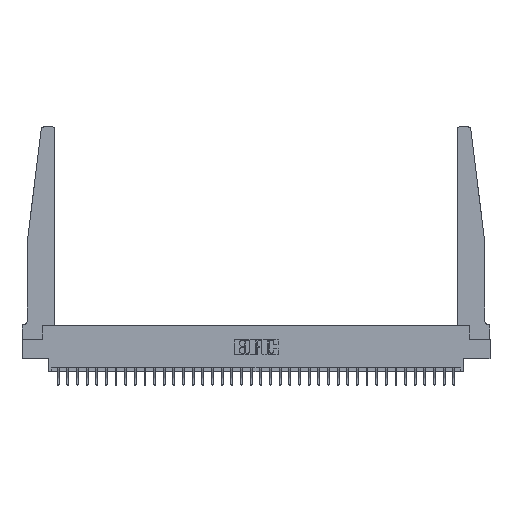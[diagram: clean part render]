
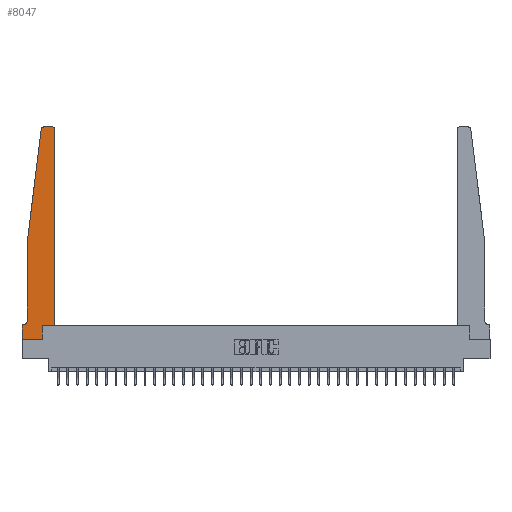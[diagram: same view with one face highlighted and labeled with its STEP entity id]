
A CAD part, top view. The second image highlights one B-rep face of the part: STEP entity #8047.
In plain terms, the highlighted planar face has unit normal (0, 0, 1).
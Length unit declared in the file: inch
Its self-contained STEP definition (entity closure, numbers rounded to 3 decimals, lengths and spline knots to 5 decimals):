
#39 = CARTESIAN_POINT ( 'NONE',  ( 0.015, 0.1875, 0.37 ) ) ;
#314 = CIRCLE ( 'NONE', #18942, 0.03 ) ;
#1138 = CARTESIAN_POINT ( 'NONE',  ( 0., 0., 0.37 ) ) ;
#1327 = CARTESIAN_POINT ( 'NONE',  ( 0.24675, 2.72367, 0.37 ) ) ;
#1437 = CARTESIAN_POINT ( 'NONE',  ( 0.25, 2.75, 0.37 ) ) ;
#2381 = DIRECTION ( 'NONE',  ( -1., 0., 0. ) ) ;
#2454 = CARTESIAN_POINT ( 'NONE',  ( 0., 0.1875, 0.37 ) ) ;
#2871 = CARTESIAN_POINT ( 'NONE',  ( 0.2605, 0.18, 0.37 ) ) ;
#2925 = ORIENTED_EDGE ( 'NONE', *, *, #31619, .T. ) ;
#3342 = VERTEX_POINT ( 'NONE', #1327 ) ;
#3439 = ORIENTED_EDGE ( 'NONE', *, *, #24675, .T. ) ;
#4040 = CARTESIAN_POINT ( 'NONE',  ( 0.425, 0.18, 0.37 ) ) ;
#4170 = ORIENTED_EDGE ( 'NONE', *, *, #29657, .T. ) ;
#4952 = VERTEX_POINT ( 'NONE', #29037 ) ;
#5104 = ORIENTED_EDGE ( 'NONE', *, *, #27729, .T. ) ;
#5352 = CARTESIAN_POINT ( 'NONE',  ( 0.015, 0.2375, 0.37 ) ) ;
#5631 = CARTESIAN_POINT ( 'NONE',  ( 0.065, 1.25, 0.37 ) ) ;
#5677 = AXIS2_PLACEMENT_3D ( 'NONE', #10539, #20381, #30613 ) ;
#5754 = CARTESIAN_POINT ( 'NONE',  ( 0.065, 1.25, 0.37 ) ) ;
#5912 = LINE ( 'NONE', #26119, #26464 ) ;
#6540 = LINE ( 'NONE', #4040, #9961 ) ;
#6696 = VECTOR ( 'NONE', #18986, 39.37008 ) ;
#6991 = VERTEX_POINT ( 'NONE', #2871 ) ;
#7453 = PLANE ( 'NONE',  #20711 ) ;
#7539 = VERTEX_POINT ( 'NONE', #30553 ) ;
#7604 = VECTOR ( 'NONE', #27082, 39.37008 ) ;
#7741 = VERTEX_POINT ( 'NONE', #18817 ) ;
#7951 = CARTESIAN_POINT ( 'NONE',  ( 0.425, 0.18, 0.37 ) ) ;
#7952 = ORIENTED_EDGE ( 'NONE', *, *, #28186, .T. ) ;
#8047 = ADVANCED_FACE ( 'NONE', ( #20122 ), #7453, .T. ) ;
#8212 = ORIENTED_EDGE ( 'NONE', *, *, #19629, .T. ) ;
#9096 = DIRECTION ( 'NONE',  ( 0., 0., 1. ) ) ;
#9371 = DIRECTION ( 'NONE',  ( 0., 1., 0. ) ) ;
#9961 = VECTOR ( 'NONE', #9371, 39.37008 ) ;
#10265 = ORIENTED_EDGE ( 'NONE', *, *, #20039, .T. ) ;
#10450 = VERTEX_POINT ( 'NONE', #32106 ) ;
#10491 = LINE ( 'NONE', #1138, #6696 ) ;
#10539 = CARTESIAN_POINT ( 'NONE',  ( 0.27653, 2.72, 0.37 ) ) ;
#11610 = DIRECTION ( 'NONE',  ( -1., 0., 0. ) ) ;
#12299 = VECTOR ( 'NONE', #2381, 39.37008 ) ;
#12859 = DIRECTION ( 'NONE',  ( 0., 0., -1. ) ) ;
#13132 = DIRECTION ( 'NONE',  ( 1., 0., 0. ) ) ;
#13327 = EDGE_CURVE ( 'NONE', #23776, #4952, #24910, .T. ) ;
#13438 = VERTEX_POINT ( 'NONE', #23059 ) ;
#13571 = ORIENTED_EDGE ( 'NONE', *, *, #19823, .T. ) ;
#13890 = CARTESIAN_POINT ( 'NONE',  ( 0., 0., 0.37 ) ) ;
#15115 = CARTESIAN_POINT ( 'NONE',  ( 0.27653, 2.75, 0.37 ) ) ;
#15221 = CARTESIAN_POINT ( 'NONE',  ( 0.065, 0.1875, 0.37 ) ) ;
#15334 = VERTEX_POINT ( 'NONE', #24056 ) ;
#16117 = VECTOR ( 'NONE', #11610, 39.37008 ) ;
#17402 = CARTESIAN_POINT ( 'NONE',  ( 0.2605, 0., 0.37 ) ) ;
#17425 = ORIENTED_EDGE ( 'NONE', *, *, #13327, .T. ) ;
#18127 = LINE ( 'NONE', #5631, #30673 ) ;
#18297 = DIRECTION ( 'NONE',  ( -0.122, -0.992, 0. ) ) ;
#18465 = LINE ( 'NONE', #7951, #22492 ) ;
#18539 = AXIS2_PLACEMENT_3D ( 'NONE', #5352, #12859, #30252 ) ;
#18580 = DIRECTION ( 'NONE',  ( 0., 1., 0. ) ) ;
#18817 = CARTESIAN_POINT ( 'NONE',  ( 0., 0., 0.37 ) ) ;
#18942 = AXIS2_PLACEMENT_3D ( 'NONE', #19432, #9096, #29997 ) ;
#18986 = DIRECTION ( 'NONE',  ( 0., -1., 0. ) ) ;
#19211 = LINE ( 'NONE', #13890, #7604 ) ;
#19432 = CARTESIAN_POINT ( 'NONE',  ( 0.395, 2.72, 0.37 ) ) ;
#19629 = EDGE_CURVE ( 'NONE', #6991, #7539, #18465, .T. ) ;
#19823 = EDGE_CURVE ( 'NONE', #10450, #30563, #24454, .T. ) ;
#20039 = EDGE_CURVE ( 'NONE', #15334, #13438, #25801, .T. ) ;
#20122 = FACE_OUTER_BOUND ( 'NONE', #27023, .T. ) ;
#20188 = VERTEX_POINT ( 'NONE', #17402 ) ;
#20381 = DIRECTION ( 'NONE',  ( 0., 0., 1. ) ) ;
#20651 = CIRCLE ( 'NONE', #18539, 0.05 ) ;
#20711 = AXIS2_PLACEMENT_3D ( 'NONE', #2454, #27846, #13132 ) ;
#21553 = ORIENTED_EDGE ( 'NONE', *, *, #27308, .T. ) ;
#21892 = EDGE_CURVE ( 'NONE', #7741, #20188, #19211, .T. ) ;
#22492 = VECTOR ( 'NONE', #26493, 39.37008 ) ;
#23059 = CARTESIAN_POINT ( 'NONE',  ( 0.065, 0.2375, 0.37 ) ) ;
#23506 = VECTOR ( 'NONE', #23761, 39.37008 ) ;
#23761 = DIRECTION ( 'NONE',  ( 0., -1., 0. ) ) ;
#23776 = VERTEX_POINT ( 'NONE', #39 ) ;
#24056 = CARTESIAN_POINT ( 'NONE',  ( 0.065, 1.25, 0.37 ) ) ;
#24454 = LINE ( 'NONE', #1437, #16117 ) ;
#24675 = EDGE_CURVE ( 'NONE', #3342, #15334, #18127, .T. ) ;
#24853 = CIRCLE ( 'NONE', #5677, 0.03 ) ;
#24910 = LINE ( 'NONE', #15221, #12299 ) ;
#25801 = LINE ( 'NONE', #5754, #23506 ) ;
#26119 = CARTESIAN_POINT ( 'NONE',  ( 0.2605, 0.18, 0.37 ) ) ;
#26464 = VECTOR ( 'NONE', #18580, 39.37008 ) ;
#26493 = DIRECTION ( 'NONE',  ( 1., 0., 0. ) ) ;
#27023 = EDGE_LOOP ( 'NONE', ( #13571, #7952, #3439, #10265, #2925, #17425, #21553, #29659, #27888, #8212, #4170, #5104 ) ) ;
#27082 = DIRECTION ( 'NONE',  ( 1., 0., 0. ) ) ;
#27308 = EDGE_CURVE ( 'NONE', #4952, #7741, #10491, .T. ) ;
#27686 = VERTEX_POINT ( 'NONE', #32160 ) ;
#27729 = EDGE_CURVE ( 'NONE', #27686, #10450, #314, .T. ) ;
#27846 = DIRECTION ( 'NONE',  ( 0., 0., 1. ) ) ;
#27888 = ORIENTED_EDGE ( 'NONE', *, *, #29128, .T. ) ;
#28186 = EDGE_CURVE ( 'NONE', #30563, #3342, #24853, .T. ) ;
#29037 = CARTESIAN_POINT ( 'NONE',  ( 0., 0.1875, 0.37 ) ) ;
#29128 = EDGE_CURVE ( 'NONE', #20188, #6991, #5912, .T. ) ;
#29657 = EDGE_CURVE ( 'NONE', #7539, #27686, #6540, .T. ) ;
#29659 = ORIENTED_EDGE ( 'NONE', *, *, #21892, .T. ) ;
#29997 = DIRECTION ( 'NONE',  ( 1., 0., 0. ) ) ;
#30252 = DIRECTION ( 'NONE',  ( -1., 0., 0. ) ) ;
#30553 = CARTESIAN_POINT ( 'NONE',  ( 0.425, 0.18, 0.37 ) ) ;
#30563 = VERTEX_POINT ( 'NONE', #15115 ) ;
#30613 = DIRECTION ( 'NONE',  ( 1., 0., 0. ) ) ;
#30673 = VECTOR ( 'NONE', #18297, 39.37008 ) ;
#31619 = EDGE_CURVE ( 'NONE', #13438, #23776, #20651, .T. ) ;
#32106 = CARTESIAN_POINT ( 'NONE',  ( 0.395, 2.75, 0.37 ) ) ;
#32160 = CARTESIAN_POINT ( 'NONE',  ( 0.425, 2.72, 0.37 ) ) ;
